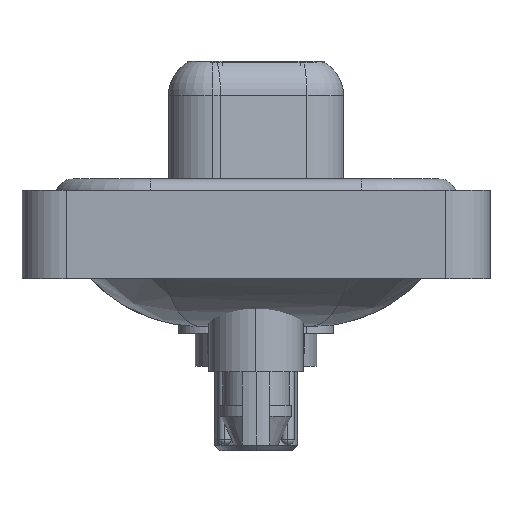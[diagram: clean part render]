
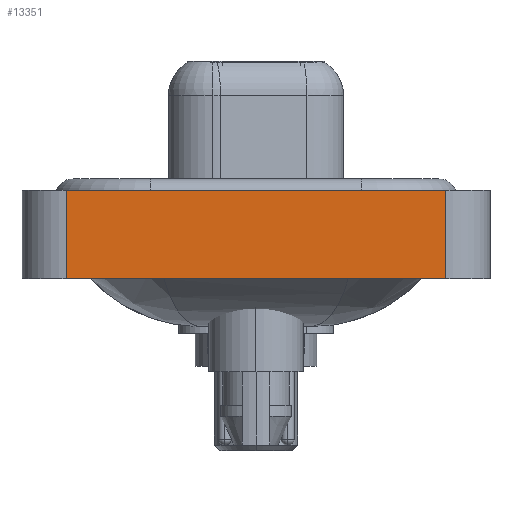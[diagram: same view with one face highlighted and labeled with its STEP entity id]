
A CAD part, left-side view. The second image highlights one B-rep face of the part: STEP entity #13351.
In plain terms, the highlighted planar face has unit normal (-1, 0, 0).
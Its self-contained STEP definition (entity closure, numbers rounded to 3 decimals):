
#501 = VECTOR ( 'NONE', #5234, 1000. ) ;
#630 = ORIENTED_EDGE ( 'NONE', *, *, #9477, .T. ) ;
#635 = VERTEX_POINT ( 'NONE', #8992 ) ;
#1301 = LINE ( 'NONE', #7627, #5707 ) ;
#2347 = LINE ( 'NONE', #13161, #501 ) ;
#2569 = DIRECTION ( 'NONE',  ( 0., -1., 0. ) ) ;
#2862 = LINE ( 'NONE', #10634, #18077 ) ;
#4128 = EDGE_CURVE ( 'NONE', #13617, #8729, #1301, .T. ) ;
#4506 = DIRECTION ( 'NONE',  ( 0., 0., 1. ) ) ;
#5234 = DIRECTION ( 'NONE',  ( 0., 0., 1. ) ) ;
#5707 = VECTOR ( 'NONE', #2569, 1000. ) ;
#6121 = VERTEX_POINT ( 'NONE', #18897 ) ;
#7358 = ORIENTED_EDGE ( 'NONE', *, *, #8796, .F. ) ;
#7516 = DIRECTION ( 'NONE',  ( 0., 0., 1. ) ) ;
#7531 = ORIENTED_EDGE ( 'NONE', *, *, #4128, .F. ) ;
#7627 = CARTESIAN_POINT ( 'NONE',  ( -7.25, -8.55, 0.4 ) ) ;
#7821 = CARTESIAN_POINT ( 'NONE',  ( -7.25, -8.55, -3.6 ) ) ;
#8006 = PLANE ( 'NONE',  #12289 ) ;
#8621 = ORIENTED_EDGE ( 'NONE', *, *, #19468, .T. ) ;
#8729 = VERTEX_POINT ( 'NONE', #8756 ) ;
#8756 = CARTESIAN_POINT ( 'NONE',  ( -7.25, -8.55, 0.4 ) ) ;
#8796 = EDGE_CURVE ( 'NONE', #6121, #13617, #2347, .T. ) ;
#8992 = CARTESIAN_POINT ( 'NONE',  ( -7.25, -8.55, -3.6 ) ) ;
#9477 = EDGE_CURVE ( 'NONE', #635, #8729, #2862, .T. ) ;
#9679 = DIRECTION ( 'NONE',  ( 0., -1., 0. ) ) ;
#10634 = CARTESIAN_POINT ( 'NONE',  ( -7.25, -8.55, -3.6 ) ) ;
#12289 = AXIS2_PLACEMENT_3D ( 'NONE', #13968, #20271, #4506 ) ;
#13077 = EDGE_LOOP ( 'NONE', ( #630, #7531, #7358, #8621 ) ) ;
#13161 = CARTESIAN_POINT ( 'NONE',  ( -7.25, 8.55, -3.6 ) ) ;
#13351 = ADVANCED_FACE ( 'NONE', ( #17550 ), #8006, .T. ) ;
#13617 = VERTEX_POINT ( 'NONE', #13753 ) ;
#13753 = CARTESIAN_POINT ( 'NONE',  ( -7.25, 8.55, 0.4 ) ) ;
#13968 = CARTESIAN_POINT ( 'NONE',  ( -7.25, -8.55, -3.6 ) ) ;
#14180 = VECTOR ( 'NONE', #9679, 1000. ) ;
#15722 = LINE ( 'NONE', #7821, #14180 ) ;
#17550 = FACE_OUTER_BOUND ( 'NONE', #13077, .T. ) ;
#18077 = VECTOR ( 'NONE', #7516, 1000. ) ;
#18897 = CARTESIAN_POINT ( 'NONE',  ( -7.25, 8.55, -3.6 ) ) ;
#19468 = EDGE_CURVE ( 'NONE', #6121, #635, #15722, .T. ) ;
#20271 = DIRECTION ( 'NONE',  ( -1., 0., 0. ) ) ;
